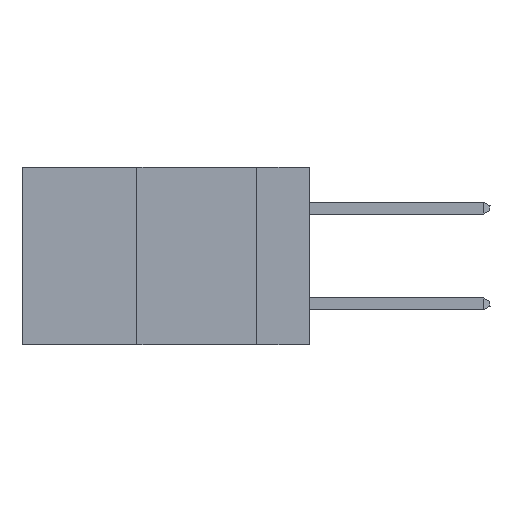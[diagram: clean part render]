
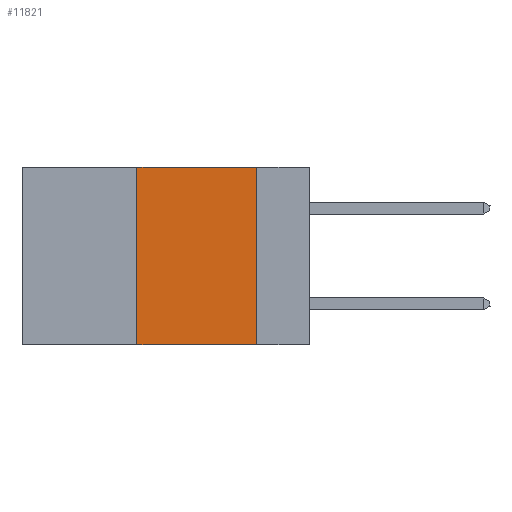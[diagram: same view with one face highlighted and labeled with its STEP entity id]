
A CAD part, left-side view. The second image highlights one B-rep face of the part: STEP entity #11821.
In plain terms, the highlighted planar face has unit normal (-1, 0, 0).
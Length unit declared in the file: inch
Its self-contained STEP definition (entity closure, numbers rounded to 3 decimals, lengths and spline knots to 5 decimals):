
#34 = VECTOR ( 'NONE', #1287, 39.37008 ) ;
#462 = EDGE_CURVE ( 'NONE', #7278, #7814, #8621, .T. ) ;
#570 = VECTOR ( 'NONE', #860, 39.37008 ) ;
#860 = DIRECTION ( 'NONE',  ( 0., 0., 1. ) ) ;
#1081 = AXIS2_PLACEMENT_3D ( 'NONE', #8678, #12539, #6769 ) ;
#1287 = DIRECTION ( 'NONE',  ( 0., -1., 0. ) ) ;
#1442 = ORIENTED_EDGE ( 'NONE', *, *, #2066, .F. ) ;
#2045 = CARTESIAN_POINT ( 'NONE',  ( 0., 0.36, 0. ) ) ;
#2063 = ORIENTED_EDGE ( 'NONE', *, *, #3567, .F. ) ;
#2066 = EDGE_CURVE ( 'NONE', #4572, #8292, #12625, .T. ) ;
#2279 = CARTESIAN_POINT ( 'NONE',  ( 0., 0.36, -0.37 ) ) ;
#2300 = EDGE_LOOP ( 'NONE', ( #1442, #2063, #8695, #6558 ) ) ;
#2651 = PLANE ( 'NONE',  #1081 ) ;
#3502 = CARTESIAN_POINT ( 'NONE',  ( 0., 0.36, 0. ) ) ;
#3567 = EDGE_CURVE ( 'NONE', #7814, #4572, #8534, .T. ) ;
#4021 = DIRECTION ( 'NONE',  ( 0., 0., -1. ) ) ;
#4572 = VERTEX_POINT ( 'NONE', #10620 ) ;
#4850 = CARTESIAN_POINT ( 'NONE',  ( 0., 0.11, -0.37 ) ) ;
#5206 = VECTOR ( 'NONE', #4021, 39.37008 ) ;
#6558 = ORIENTED_EDGE ( 'NONE', *, *, #10348, .T. ) ;
#6769 = DIRECTION ( 'NONE',  ( 0., 0., -1. ) ) ;
#7128 = CARTESIAN_POINT ( 'NONE',  ( 0., 0.6, 0. ) ) ;
#7278 = VERTEX_POINT ( 'NONE', #2279 ) ;
#7814 = VERTEX_POINT ( 'NONE', #2045 ) ;
#8292 = VERTEX_POINT ( 'NONE', #4850 ) ;
#8534 = LINE ( 'NONE', #7128, #10801 ) ;
#8621 = LINE ( 'NONE', #3502, #570 ) ;
#8678 = CARTESIAN_POINT ( 'NONE',  ( 0., 0.6, 0. ) ) ;
#8695 = ORIENTED_EDGE ( 'NONE', *, *, #462, .F. ) ;
#9333 = FACE_OUTER_BOUND ( 'NONE', #2300, .T. ) ;
#10243 = CARTESIAN_POINT ( 'NONE',  ( 0., 0.6, -0.37 ) ) ;
#10348 = EDGE_CURVE ( 'NONE', #7278, #8292, #10995, .T. ) ;
#10620 = CARTESIAN_POINT ( 'NONE',  ( 0., 0.11, 0. ) ) ;
#10801 = VECTOR ( 'NONE', #11932, 39.37008 ) ;
#10923 = CARTESIAN_POINT ( 'NONE',  ( 0., 0.11, 0. ) ) ;
#10995 = LINE ( 'NONE', #10243, #34 ) ;
#11821 = ADVANCED_FACE ( 'NONE', ( #9333 ), #2651, .F. ) ;
#11932 = DIRECTION ( 'NONE',  ( 0., -1., 0. ) ) ;
#12539 = DIRECTION ( 'NONE',  ( 1., 0., 0. ) ) ;
#12625 = LINE ( 'NONE', #10923, #5206 ) ;
